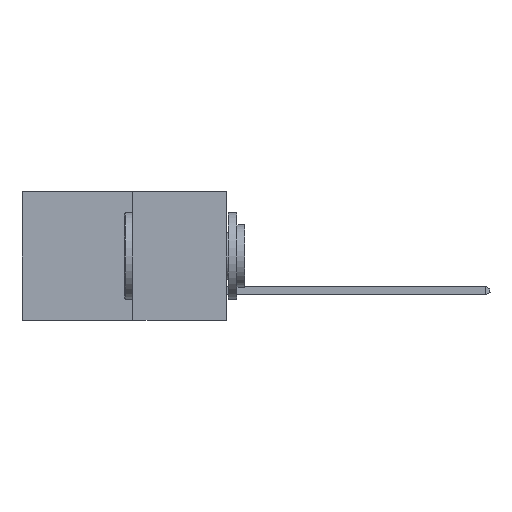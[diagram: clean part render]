
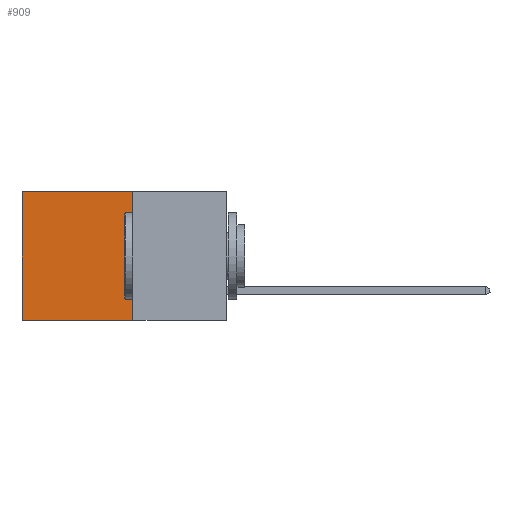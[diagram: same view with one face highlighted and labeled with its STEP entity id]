
A CAD part, left-side view. The second image highlights one B-rep face of the part: STEP entity #909.
In plain terms, the highlighted planar face has unit normal (-1, 0, 0).
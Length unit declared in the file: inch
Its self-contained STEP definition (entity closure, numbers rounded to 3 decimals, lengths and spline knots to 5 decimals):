
#523 = DIRECTION ( 'NONE',  ( 0., 0., -1. ) ) ;
#909 = ADVANCED_FACE ( 'NONE', ( #3318 ), #2083, .F. ) ;
#2083 = PLANE ( 'NONE',  #13140 ) ;
#2140 = CARTESIAN_POINT ( 'NONE',  ( 0.277, 0.27, 0. ) ) ;
#2169 = VECTOR ( 'NONE', #12173, 39.37008 ) ;
#3318 = FACE_OUTER_BOUND ( 'NONE', #10294, .T. ) ;
#4254 = ORIENTED_EDGE ( 'NONE', *, *, #13312, .F. ) ;
#4489 = LINE ( 'NONE', #9872, #7320 ) ;
#4767 = EDGE_CURVE ( 'NONE', #9317, #11321, #4489, .T. ) ;
#5030 = LINE ( 'NONE', #11204, #2169 ) ;
#5105 = VECTOR ( 'NONE', #12396, 39.37008 ) ;
#5467 = DIRECTION ( 'NONE',  ( 0., 0., -1. ) ) ;
#6075 = ORIENTED_EDGE ( 'NONE', *, *, #4767, .F. ) ;
#6082 = LINE ( 'NONE', #13179, #8242 ) ;
#6744 = EDGE_CURVE ( 'NONE', #12187, #10054, #10985, .T. ) ;
#7192 = EDGE_CURVE ( 'NONE', #10054, #11321, #6082, .T. ) ;
#7320 = VECTOR ( 'NONE', #12834, 39.37008 ) ;
#7907 = DIRECTION ( 'NONE',  ( 1., 0., 0. ) ) ;
#8242 = VECTOR ( 'NONE', #523, 39.37008 ) ;
#8343 = CARTESIAN_POINT ( 'NONE',  ( 0.277, 0.27, 0. ) ) ;
#8819 = CARTESIAN_POINT ( 'NONE',  ( 0.277, 0.59, 0. ) ) ;
#9317 = VERTEX_POINT ( 'NONE', #11799 ) ;
#9872 = CARTESIAN_POINT ( 'NONE',  ( 0.277, 0.27, -0.37 ) ) ;
#10054 = VERTEX_POINT ( 'NONE', #8819 ) ;
#10294 = EDGE_LOOP ( 'NONE', ( #10496, #6075, #4254, #12496 ) ) ;
#10496 = ORIENTED_EDGE ( 'NONE', *, *, #7192, .T. ) ;
#10985 = LINE ( 'NONE', #8343, #5105 ) ;
#11204 = CARTESIAN_POINT ( 'NONE',  ( 0.277, 0.27, -0.37 ) ) ;
#11321 = VERTEX_POINT ( 'NONE', #12341 ) ;
#11799 = CARTESIAN_POINT ( 'NONE',  ( 0.277, 0.27, -0.37 ) ) ;
#12173 = DIRECTION ( 'NONE',  ( 0., 0., -1. ) ) ;
#12187 = VERTEX_POINT ( 'NONE', #2140 ) ;
#12341 = CARTESIAN_POINT ( 'NONE',  ( 0.277, 0.59, -0.37 ) ) ;
#12396 = DIRECTION ( 'NONE',  ( 0., 1., 0. ) ) ;
#12496 = ORIENTED_EDGE ( 'NONE', *, *, #6744, .T. ) ;
#12834 = DIRECTION ( 'NONE',  ( 0., 1., 0. ) ) ;
#12948 = CARTESIAN_POINT ( 'NONE',  ( 0.277, 0.27, -0.37 ) ) ;
#13140 = AXIS2_PLACEMENT_3D ( 'NONE', #12948, #7907, #5467 ) ;
#13179 = CARTESIAN_POINT ( 'NONE',  ( 0.277, 0.59, -0.37 ) ) ;
#13312 = EDGE_CURVE ( 'NONE', #12187, #9317, #5030, .T. ) ;
